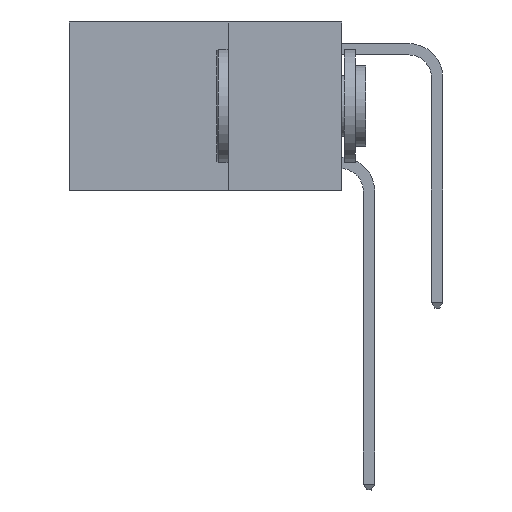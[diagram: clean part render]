
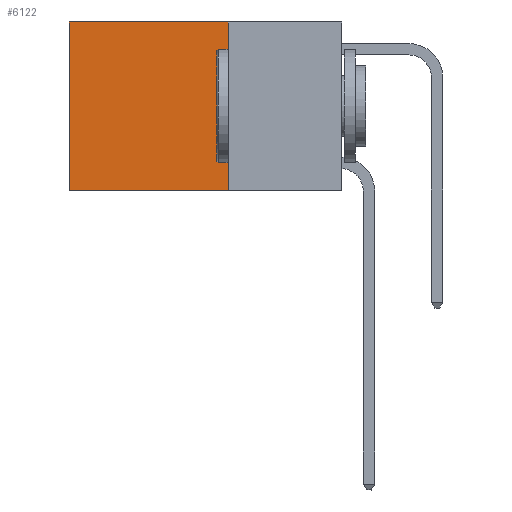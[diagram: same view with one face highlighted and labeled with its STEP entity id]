
A CAD part, left-side view. The second image highlights one B-rep face of the part: STEP entity #6122.
In plain terms, the highlighted planar face has unit normal (-1, 0, 0).
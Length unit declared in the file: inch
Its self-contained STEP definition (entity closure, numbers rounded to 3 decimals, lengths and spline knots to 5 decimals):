
#249 = EDGE_CURVE ( 'NONE', #923, #23100, #13112, .T. ) ;
#351 = PLANE ( 'NONE',  #10189 ) ;
#923 = VERTEX_POINT ( 'NONE', #21884 ) ;
#1822 = CARTESIAN_POINT ( 'NONE',  ( 0.2625, 0.25, -0.37 ) ) ;
#1992 = DIRECTION ( 'NONE',  ( 0., 0., -1. ) ) ;
#2298 = DIRECTION ( 'NONE',  ( 1., 0., 0. ) ) ;
#3172 = VECTOR ( 'NONE', #4595, 39.37008 ) ;
#3255 = CARTESIAN_POINT ( 'NONE',  ( 0.2625, 0.6, 0. ) ) ;
#3389 = VECTOR ( 'NONE', #16297, 39.37008 ) ;
#4595 = DIRECTION ( 'NONE',  ( 0., 0., -1. ) ) ;
#5070 = VERTEX_POINT ( 'NONE', #10160 ) ;
#5766 = CARTESIAN_POINT ( 'NONE',  ( 0.2625, 0.25, 0. ) ) ;
#6122 = ADVANCED_FACE ( 'NONE', ( #20985 ), #351, .F. ) ;
#7081 = CARTESIAN_POINT ( 'NONE',  ( 0.2625, 0.25, 0. ) ) ;
#7446 = ORIENTED_EDGE ( 'NONE', *, *, #249, .T. ) ;
#7849 = CARTESIAN_POINT ( 'NONE',  ( 0.2625, 0.25, 0. ) ) ;
#8214 = VECTOR ( 'NONE', #1992, 39.37008 ) ;
#10160 = CARTESIAN_POINT ( 'NONE',  ( 0.2625, 0.25, 0. ) ) ;
#10189 = AXIS2_PLACEMENT_3D ( 'NONE', #7849, #2298, #15376 ) ;
#11627 = EDGE_CURVE ( 'NONE', #5070, #923, #13321, .T. ) ;
#13112 = LINE ( 'NONE', #3255, #3172 ) ;
#13321 = LINE ( 'NONE', #7081, #3389 ) ;
#13849 = CARTESIAN_POINT ( 'NONE',  ( 0.2625, 0.25, -0.37 ) ) ;
#15376 = DIRECTION ( 'NONE',  ( 0., 0., -1. ) ) ;
#16297 = DIRECTION ( 'NONE',  ( 0., 1., 0. ) ) ;
#17459 = CARTESIAN_POINT ( 'NONE',  ( 0.2625, 0.6, -0.37 ) ) ;
#17802 = VECTOR ( 'NONE', #21294, 39.37008 ) ;
#17959 = ORIENTED_EDGE ( 'NONE', *, *, #20855, .F. ) ;
#18696 = LINE ( 'NONE', #5766, #8214 ) ;
#18836 = ORIENTED_EDGE ( 'NONE', *, *, #11627, .T. ) ;
#20855 = EDGE_CURVE ( 'NONE', #5070, #22852, #18696, .T. ) ;
#20985 = FACE_OUTER_BOUND ( 'NONE', #21283, .T. ) ;
#21067 = EDGE_CURVE ( 'NONE', #22852, #23100, #22769, .T. ) ;
#21283 = EDGE_LOOP ( 'NONE', ( #7446, #21396, #17959, #18836 ) ) ;
#21294 = DIRECTION ( 'NONE',  ( 0., 1., 0. ) ) ;
#21396 = ORIENTED_EDGE ( 'NONE', *, *, #21067, .F. ) ;
#21884 = CARTESIAN_POINT ( 'NONE',  ( 0.2625, 0.6, 0. ) ) ;
#22769 = LINE ( 'NONE', #13849, #17802 ) ;
#22852 = VERTEX_POINT ( 'NONE', #1822 ) ;
#23100 = VERTEX_POINT ( 'NONE', #17459 ) ;
